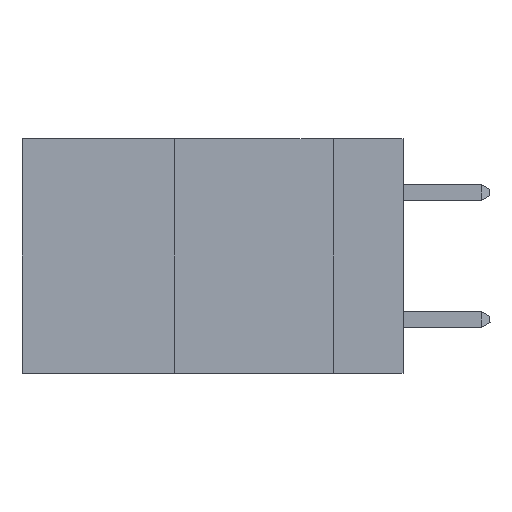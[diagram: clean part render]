
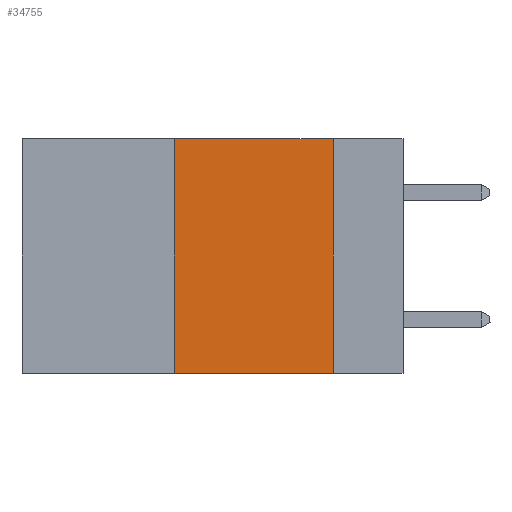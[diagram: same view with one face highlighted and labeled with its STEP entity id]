
A CAD part, left-side view. The second image highlights one B-rep face of the part: STEP entity #34755.
In plain terms, the highlighted planar face has unit normal (-1, 0, 0).
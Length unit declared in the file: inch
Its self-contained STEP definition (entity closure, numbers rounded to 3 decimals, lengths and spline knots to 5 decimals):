
#499 = DIRECTION ( 'NONE',  ( 0., -1., 0. ) ) ;
#1270 = ORIENTED_EDGE ( 'NONE', *, *, #8814, .F. ) ;
#4060 = DIRECTION ( 'NONE',  ( 0., -1., 0. ) ) ;
#4624 = VECTOR ( 'NONE', #31760, 39.37008 ) ;
#5209 = VERTEX_POINT ( 'NONE', #17259 ) ;
#6498 = VERTEX_POINT ( 'NONE', #27780 ) ;
#8814 = EDGE_CURVE ( 'NONE', #34374, #18459, #37746, .T. ) ;
#11260 = EDGE_CURVE ( 'NONE', #5209, #6498, #36554, .T. ) ;
#11358 = CARTESIAN_POINT ( 'NONE',  ( 0., 0.36, 0. ) ) ;
#12860 = DIRECTION ( 'NONE',  ( 1., 0., 0. ) ) ;
#15194 = LINE ( 'NONE', #37199, #4624 ) ;
#16488 = CARTESIAN_POINT ( 'NONE',  ( 0., 0.11, 0. ) ) ;
#16506 = CARTESIAN_POINT ( 'NONE',  ( 0., 0.6, 0. ) ) ;
#17259 = CARTESIAN_POINT ( 'NONE',  ( 0., 0.36, -0.37 ) ) ;
#17417 = ORIENTED_EDGE ( 'NONE', *, *, #37341, .F. ) ;
#18459 = VERTEX_POINT ( 'NONE', #22834 ) ;
#18867 = ORIENTED_EDGE ( 'NONE', *, *, #11260, .T. ) ;
#20159 = VECTOR ( 'NONE', #499, 39.37008 ) ;
#22552 = DIRECTION ( 'NONE',  ( 0., 0., -1. ) ) ;
#22834 = CARTESIAN_POINT ( 'NONE',  ( 0., 0.11, 0. ) ) ;
#22914 = FACE_OUTER_BOUND ( 'NONE', #37944, .T. ) ;
#26968 = CARTESIAN_POINT ( 'NONE',  ( 0., 0.6, -0.37 ) ) ;
#27780 = CARTESIAN_POINT ( 'NONE',  ( 0., 0.11, -0.37 ) ) ;
#29285 = EDGE_CURVE ( 'NONE', #18459, #6498, #39399, .T. ) ;
#31760 = DIRECTION ( 'NONE',  ( 0., 0., 1. ) ) ;
#32283 = PLANE ( 'NONE',  #35064 ) ;
#32555 = CARTESIAN_POINT ( 'NONE',  ( 0., 0.6, 0. ) ) ;
#33182 = ORIENTED_EDGE ( 'NONE', *, *, #29285, .F. ) ;
#34374 = VERTEX_POINT ( 'NONE', #11358 ) ;
#34755 = ADVANCED_FACE ( 'NONE', ( #22914 ), #32283, .F. ) ;
#35054 = VECTOR ( 'NONE', #4060, 39.37008 ) ;
#35064 = AXIS2_PLACEMENT_3D ( 'NONE', #16506, #12860, #22552 ) ;
#35885 = DIRECTION ( 'NONE',  ( 0., 0., -1. ) ) ;
#36554 = LINE ( 'NONE', #26968, #35054 ) ;
#37199 = CARTESIAN_POINT ( 'NONE',  ( 0., 0.36, 0. ) ) ;
#37341 = EDGE_CURVE ( 'NONE', #5209, #34374, #15194, .T. ) ;
#37746 = LINE ( 'NONE', #32555, #20159 ) ;
#37944 = EDGE_LOOP ( 'NONE', ( #33182, #1270, #17417, #18867 ) ) ;
#38909 = VECTOR ( 'NONE', #35885, 39.37008 ) ;
#39399 = LINE ( 'NONE', #16488, #38909 ) ;
